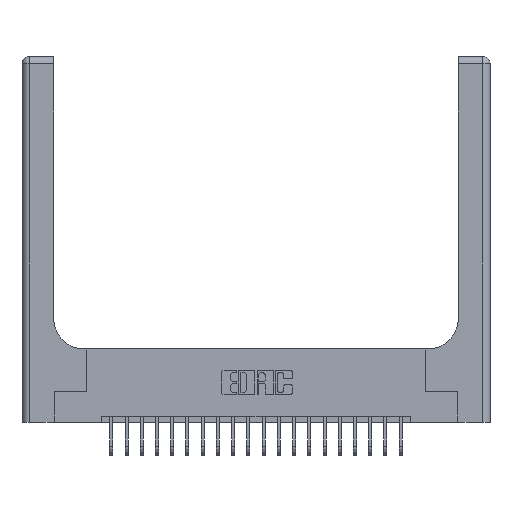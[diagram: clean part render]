
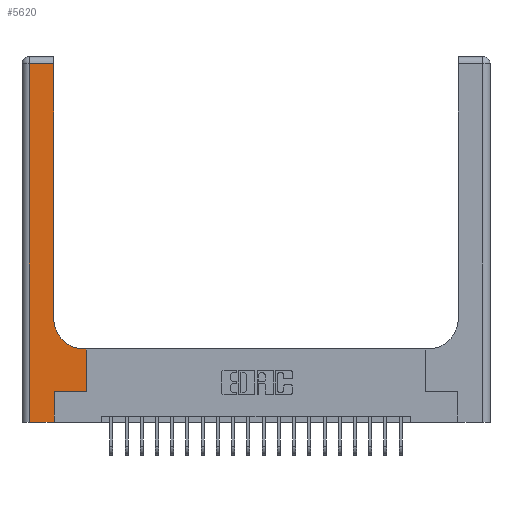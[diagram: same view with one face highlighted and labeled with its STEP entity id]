
A CAD part, top view. The second image highlights one B-rep face of the part: STEP entity #5620.
In plain terms, the highlighted planar face has unit normal (0, 0, 1).
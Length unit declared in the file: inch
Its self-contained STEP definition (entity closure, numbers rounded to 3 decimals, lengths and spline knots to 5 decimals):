
#62 = DIRECTION ( 'NONE',  ( 1., 0., 0. ) ) ;
#276 = CARTESIAN_POINT ( 'NONE',  ( 0.26, 0.6, 0.37 ) ) ;
#394 = ORIENTED_EDGE ( 'NONE', *, *, #4991, .T. ) ;
#399 = EDGE_CURVE ( 'NONE', #2787, #19177, #689, .T. ) ;
#689 = LINE ( 'NONE', #7910, #11006 ) ;
#808 = VERTEX_POINT ( 'NONE', #19603 ) ;
#937 = FACE_OUTER_BOUND ( 'NONE', #17519, .T. ) ;
#977 = CARTESIAN_POINT ( 'NONE',  ( 0.265, 0.25, 0.37 ) ) ;
#1608 = CARTESIAN_POINT ( 'NONE',  ( 0.528, 0.25, 0.37 ) ) ;
#1963 = CIRCLE ( 'NONE', #3086, 0.25 ) ;
#2089 = CARTESIAN_POINT ( 'NONE',  ( 0.265, 0.25, 0.37 ) ) ;
#2586 = VECTOR ( 'NONE', #14724, 39.37008 ) ;
#2787 = VERTEX_POINT ( 'NONE', #17801 ) ;
#2956 = PLANE ( 'NONE',  #10703 ) ;
#3086 = AXIS2_PLACEMENT_3D ( 'NONE', #3749, #13107, #62 ) ;
#3490 = DIRECTION ( 'NONE',  ( 0., 1., 0. ) ) ;
#3749 = CARTESIAN_POINT ( 'NONE',  ( 0.51, 0.85, 0.37 ) ) ;
#4840 = VECTOR ( 'NONE', #5984, 39.37008 ) ;
#4991 = EDGE_CURVE ( 'NONE', #9289, #21068, #1963, .T. ) ;
#5133 = VERTEX_POINT ( 'NONE', #18802 ) ;
#5620 = ADVANCED_FACE ( 'NONE', ( #937 ), #2956, .F. ) ;
#5984 = DIRECTION ( 'NONE',  ( 1., 0., 0. ) ) ;
#6020 = DIRECTION ( 'NONE',  ( 0., 1., 0. ) ) ;
#6247 = EDGE_CURVE ( 'NONE', #5133, #18173, #12495, .T. ) ;
#6491 = DIRECTION ( 'NONE',  ( -1., 0., 0. ) ) ;
#6921 = CARTESIAN_POINT ( 'NONE',  ( 0.51, 0.6, 0.37 ) ) ;
#6949 = ORIENTED_EDGE ( 'NONE', *, *, #14277, .T. ) ;
#7751 = LINE ( 'NONE', #2089, #4840 ) ;
#7906 = DIRECTION ( 'NONE',  ( -1., 0., 0. ) ) ;
#7910 = CARTESIAN_POINT ( 'NONE',  ( 0.06, 3., 0.37 ) ) ;
#8053 = VERTEX_POINT ( 'NONE', #1608 ) ;
#8275 = CARTESIAN_POINT ( 'NONE',  ( 0., 3., 0.37 ) ) ;
#8592 = EDGE_CURVE ( 'NONE', #21068, #808, #21816, .T. ) ;
#9147 = VECTOR ( 'NONE', #7906, 39.37008 ) ;
#9289 = VERTEX_POINT ( 'NONE', #6921 ) ;
#9391 = EDGE_CURVE ( 'NONE', #23279, #9289, #12851, .T. ) ;
#9506 = DIRECTION ( 'NONE',  ( -1., 0., 0. ) ) ;
#10703 = AXIS2_PLACEMENT_3D ( 'NONE', #8275, #15501, #6491 ) ;
#10707 = DIRECTION ( 'NONE',  ( 0., 1., 0. ) ) ;
#11006 = VECTOR ( 'NONE', #15136, 39.37008 ) ;
#11388 = ORIENTED_EDGE ( 'NONE', *, *, #19023, .T. ) ;
#12247 = CARTESIAN_POINT ( 'NONE',  ( 0.528, 0.25, 0.37 ) ) ;
#12495 = LINE ( 'NONE', #19729, #14483 ) ;
#12615 = ORIENTED_EDGE ( 'NONE', *, *, #8592, .T. ) ;
#12681 = VECTOR ( 'NONE', #10707, 39.37008 ) ;
#12851 = LINE ( 'NONE', #276, #14145 ) ;
#13107 = DIRECTION ( 'NONE',  ( 0., 0., -1. ) ) ;
#13347 = CARTESIAN_POINT ( 'NONE',  ( 0.528, 0.6, 0.37 ) ) ;
#13474 = CARTESIAN_POINT ( 'NONE',  ( 0., 2.94, 0.37 ) ) ;
#13907 = LINE ( 'NONE', #12247, #12681 ) ;
#14145 = VECTOR ( 'NONE', #9506, 39.37008 ) ;
#14186 = VECTOR ( 'NONE', #6020, 39.37008 ) ;
#14277 = EDGE_CURVE ( 'NONE', #18173, #8053, #7751, .T. ) ;
#14483 = VECTOR ( 'NONE', #3490, 39.37008 ) ;
#14488 = LINE ( 'NONE', #16746, #2586 ) ;
#14681 = EDGE_CURVE ( 'NONE', #19177, #5133, #14488, .T. ) ;
#14724 = DIRECTION ( 'NONE',  ( 1., 0., 0. ) ) ;
#15136 = DIRECTION ( 'NONE',  ( 0., -1., 0. ) ) ;
#15501 = DIRECTION ( 'NONE',  ( 0., 0., -1. ) ) ;
#15592 = ORIENTED_EDGE ( 'NONE', *, *, #9391, .T. ) ;
#15781 = ORIENTED_EDGE ( 'NONE', *, *, #22472, .T. ) ;
#16205 = ORIENTED_EDGE ( 'NONE', *, *, #14681, .T. ) ;
#16258 = ORIENTED_EDGE ( 'NONE', *, *, #399, .T. ) ;
#16746 = CARTESIAN_POINT ( 'NONE',  ( 0., 0., 0.37 ) ) ;
#17519 = EDGE_LOOP ( 'NONE', ( #12615, #11388, #16258, #16205, #18521, #6949, #15781, #15592, #394 ) ) ;
#17801 = CARTESIAN_POINT ( 'NONE',  ( 0.06, 2.94, 0.37 ) ) ;
#18173 = VERTEX_POINT ( 'NONE', #977 ) ;
#18246 = CARTESIAN_POINT ( 'NONE',  ( 0.26, 3., 0.37 ) ) ;
#18521 = ORIENTED_EDGE ( 'NONE', *, *, #6247, .T. ) ;
#18554 = CARTESIAN_POINT ( 'NONE',  ( 0.26, 0.85, 0.37 ) ) ;
#18802 = CARTESIAN_POINT ( 'NONE',  ( 0.265, 0., 0.37 ) ) ;
#19023 = EDGE_CURVE ( 'NONE', #808, #2787, #22386, .T. ) ;
#19177 = VERTEX_POINT ( 'NONE', #20496 ) ;
#19603 = CARTESIAN_POINT ( 'NONE',  ( 0.26, 2.94, 0.37 ) ) ;
#19729 = CARTESIAN_POINT ( 'NONE',  ( 0.265, 0., 0.37 ) ) ;
#20496 = CARTESIAN_POINT ( 'NONE',  ( 0.06, 0., 0.37 ) ) ;
#21068 = VERTEX_POINT ( 'NONE', #18554 ) ;
#21816 = LINE ( 'NONE', #18246, #14186 ) ;
#22386 = LINE ( 'NONE', #13474, #9147 ) ;
#22472 = EDGE_CURVE ( 'NONE', #8053, #23279, #13907, .T. ) ;
#23279 = VERTEX_POINT ( 'NONE', #13347 ) ;
